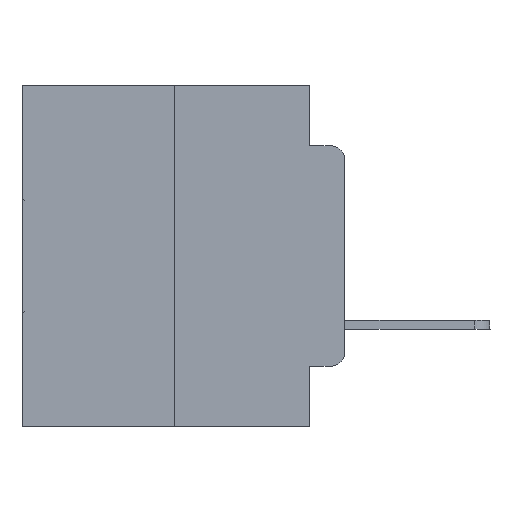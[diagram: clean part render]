
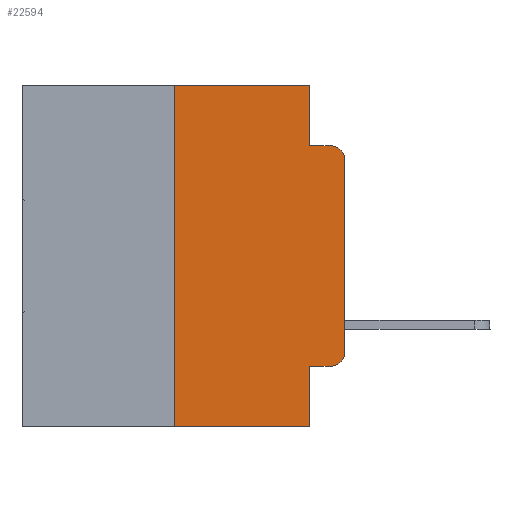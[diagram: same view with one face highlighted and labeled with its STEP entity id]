
A CAD part, left-side view. The second image highlights one B-rep face of the part: STEP entity #22594.
In plain terms, the highlighted planar face has unit normal (-1, 0, 0).
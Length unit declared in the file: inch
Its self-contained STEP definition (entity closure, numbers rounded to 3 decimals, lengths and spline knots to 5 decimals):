
#183 = VECTOR ( 'NONE', #4949, 39.37008 ) ;
#601 = ORIENTED_EDGE ( 'NONE', *, *, #19694, .T. ) ;
#843 = EDGE_LOOP ( 'NONE', ( #26616, #8657, #18611, #26450, #18958, #19784, #3323, #26223, #601, #19958 ) ) ;
#1704 = CARTESIAN_POINT ( 'NONE',  ( 0., 0.02, -0.3915 ) ) ;
#2474 = LINE ( 'NONE', #9617, #2987 ) ;
#2687 = VECTOR ( 'NONE', #11265, 39.37008 ) ;
#2921 = DIRECTION ( 'NONE',  ( 0., -1., 0. ) ) ;
#2987 = VECTOR ( 'NONE', #16536, 39.37008 ) ;
#3323 = ORIENTED_EDGE ( 'NONE', *, *, #19259, .T. ) ;
#4567 = CARTESIAN_POINT ( 'NONE',  ( 0., 0.25, -0.5 ) ) ;
#4847 = VECTOR ( 'NONE', #25958, 39.37008 ) ;
#4949 = DIRECTION ( 'NONE',  ( 0., -1., 0. ) ) ;
#5024 = DIRECTION ( 'NONE',  ( 0., -1., 0. ) ) ;
#5241 = LINE ( 'NONE', #14670, #20540 ) ;
#6491 = CARTESIAN_POINT ( 'NONE',  ( 0., 0.051, -0.0885 ) ) ;
#7307 = CARTESIAN_POINT ( 'NONE',  ( 0., 0.051, 0. ) ) ;
#7439 = CARTESIAN_POINT ( 'NONE',  ( 0., 0.473, -0.5 ) ) ;
#7480 = DIRECTION ( 'NONE',  ( 0., 0., -1. ) ) ;
#7522 = DIRECTION ( 'NONE',  ( 0., 0., 1. ) ) ;
#7646 = CARTESIAN_POINT ( 'NONE',  ( 0., 0., -0.3915 ) ) ;
#8164 = VECTOR ( 'NONE', #15447, 39.37008 ) ;
#8657 = ORIENTED_EDGE ( 'NONE', *, *, #23042, .T. ) ;
#8890 = VERTEX_POINT ( 'NONE', #21090 ) ;
#9148 = CARTESIAN_POINT ( 'NONE',  ( 0., 0., -0.1085 ) ) ;
#9217 = AXIS2_PLACEMENT_3D ( 'NONE', #1704, #11152, #20574 ) ;
#9457 = EDGE_CURVE ( 'NONE', #9866, #17837, #5241, .T. ) ;
#9557 = VERTEX_POINT ( 'NONE', #29957 ) ;
#9617 = CARTESIAN_POINT ( 'NONE',  ( 0., 0.051, 0. ) ) ;
#9866 = VERTEX_POINT ( 'NONE', #21749 ) ;
#10442 = LINE ( 'NONE', #17535, #12665 ) ;
#10943 = VERTEX_POINT ( 'NONE', #6491 ) ;
#11152 = DIRECTION ( 'NONE',  ( -1., 0., 0. ) ) ;
#11265 = DIRECTION ( 'NONE',  ( 0., -1., 0. ) ) ;
#12452 = DIRECTION ( 'NONE',  ( 0., 0., -1. ) ) ;
#12606 = DIRECTION ( 'NONE',  ( 1., 0., 0. ) ) ;
#12665 = VECTOR ( 'NONE', #5024, 39.37008 ) ;
#13622 = CARTESIAN_POINT ( 'NONE',  ( 0., 0., 0. ) ) ;
#13664 = VERTEX_POINT ( 'NONE', #4567 ) ;
#13730 = LINE ( 'NONE', #15877, #2687 ) ;
#14135 = VERTEX_POINT ( 'NONE', #9148 ) ;
#14153 = EDGE_CURVE ( 'NONE', #9557, #15066, #2474, .T. ) ;
#14317 = VERTEX_POINT ( 'NONE', #19329 ) ;
#14606 = AXIS2_PLACEMENT_3D ( 'NONE', #17079, #12606, #12452 ) ;
#14670 = CARTESIAN_POINT ( 'NONE',  ( 0., 0.473, 0. ) ) ;
#15066 = VERTEX_POINT ( 'NONE', #23122 ) ;
#15447 = DIRECTION ( 'NONE',  ( 0., 0., -1. ) ) ;
#15877 = CARTESIAN_POINT ( 'NONE',  ( 0., 0.051, -0.4115 ) ) ;
#16536 = DIRECTION ( 'NONE',  ( 0., 0., -1. ) ) ;
#17079 = CARTESIAN_POINT ( 'NONE',  ( 0., 0.473, 0. ) ) ;
#17535 = CARTESIAN_POINT ( 'NONE',  ( 0., 0.051, -0.0885 ) ) ;
#17542 = LINE ( 'NONE', #23892, #19462 ) ;
#17837 = VERTEX_POINT ( 'NONE', #7307 ) ;
#18611 = ORIENTED_EDGE ( 'NONE', *, *, #22621, .F. ) ;
#18666 = AXIS2_PLACEMENT_3D ( 'NONE', #26637, #28652, #7480 ) ;
#18958 = ORIENTED_EDGE ( 'NONE', *, *, #9457, .F. ) ;
#19259 = EDGE_CURVE ( 'NONE', #13664, #15066, #26134, .T. ) ;
#19329 = CARTESIAN_POINT ( 'NONE',  ( 0., 0.02, -0.0885 ) ) ;
#19401 = FACE_OUTER_BOUND ( 'NONE', #843, .T. ) ;
#19462 = VECTOR ( 'NONE', #7522, 39.37008 ) ;
#19694 = EDGE_CURVE ( 'NONE', #9557, #8890, #13730, .T. ) ;
#19784 = ORIENTED_EDGE ( 'NONE', *, *, #26095, .F. ) ;
#19958 = ORIENTED_EDGE ( 'NONE', *, *, #21528, .T. ) ;
#20540 = VECTOR ( 'NONE', #2921, 39.37008 ) ;
#20574 = DIRECTION ( 'NONE',  ( 0., 0., -1. ) ) ;
#21090 = CARTESIAN_POINT ( 'NONE',  ( 0., 0.02, -0.4115 ) ) ;
#21159 = LINE ( 'NONE', #13622, #4847 ) ;
#21528 = EDGE_CURVE ( 'NONE', #8890, #27844, #22539, .T. ) ;
#21749 = CARTESIAN_POINT ( 'NONE',  ( 0., 0.25, 0. ) ) ;
#21871 = PLANE ( 'NONE',  #14606 ) ;
#22539 = CIRCLE ( 'NONE', #9217, 0.02 ) ;
#22594 = ADVANCED_FACE ( 'NONE', ( #19401 ), #21871, .F. ) ;
#22621 = EDGE_CURVE ( 'NONE', #10943, #14317, #10442, .T. ) ;
#23042 = EDGE_CURVE ( 'NONE', #14135, #14317, #27562, .T. ) ;
#23122 = CARTESIAN_POINT ( 'NONE',  ( 0., 0.051, -0.5 ) ) ;
#23368 = EDGE_CURVE ( 'NONE', #27844, #14135, #21159, .T. ) ;
#23892 = CARTESIAN_POINT ( 'NONE',  ( 0., 0.25, 0. ) ) ;
#24575 = LINE ( 'NONE', #26911, #8164 ) ;
#25958 = DIRECTION ( 'NONE',  ( 0., 0., 1. ) ) ;
#26095 = EDGE_CURVE ( 'NONE', #13664, #9866, #17542, .T. ) ;
#26134 = LINE ( 'NONE', #7439, #183 ) ;
#26223 = ORIENTED_EDGE ( 'NONE', *, *, #14153, .F. ) ;
#26450 = ORIENTED_EDGE ( 'NONE', *, *, #28400, .F. ) ;
#26616 = ORIENTED_EDGE ( 'NONE', *, *, #23368, .T. ) ;
#26637 = CARTESIAN_POINT ( 'NONE',  ( 0., 0.02, -0.1085 ) ) ;
#26911 = CARTESIAN_POINT ( 'NONE',  ( 0., 0.051, 0. ) ) ;
#27562 = CIRCLE ( 'NONE', #18666, 0.02 ) ;
#27844 = VERTEX_POINT ( 'NONE', #7646 ) ;
#28400 = EDGE_CURVE ( 'NONE', #17837, #10943, #24575, .T. ) ;
#28652 = DIRECTION ( 'NONE',  ( -1., 0., 0. ) ) ;
#29957 = CARTESIAN_POINT ( 'NONE',  ( 0., 0.051, -0.4115 ) ) ;
